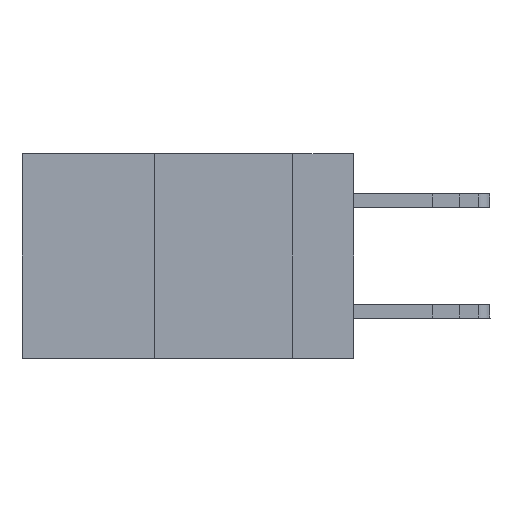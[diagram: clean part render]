
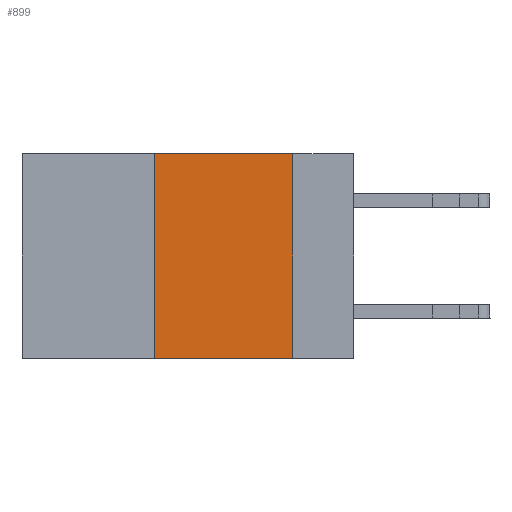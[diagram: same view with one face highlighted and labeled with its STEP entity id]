
A CAD part, left-side view. The second image highlights one B-rep face of the part: STEP entity #899.
In plain terms, the highlighted planar face has unit normal (-1, 0, 0).
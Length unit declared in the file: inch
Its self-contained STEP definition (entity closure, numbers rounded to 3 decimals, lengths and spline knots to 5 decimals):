
#395 = CARTESIAN_POINT ( 'NONE',  ( 0., 0.11, 0. ) ) ;
#654 = VERTEX_POINT ( 'NONE', #395 ) ;
#899 = ADVANCED_FACE ( 'NONE', ( #26525 ), #13610, .F. ) ;
#933 = EDGE_CURVE ( 'NONE', #654, #10693, #12890, .T. ) ;
#2144 = DIRECTION ( 'NONE',  ( 0., 0., -1. ) ) ;
#2252 = VERTEX_POINT ( 'NONE', #13262 ) ;
#3019 = LINE ( 'NONE', #32753, #29172 ) ;
#3644 = DIRECTION ( 'NONE',  ( 0., 0., 1. ) ) ;
#4279 = CARTESIAN_POINT ( 'NONE',  ( 0., 0.36, -0.37 ) ) ;
#5188 = CARTESIAN_POINT ( 'NONE',  ( 0., 0.6, 0. ) ) ;
#7033 = ORIENTED_EDGE ( 'NONE', *, *, #8444, .T. ) ;
#7741 = CARTESIAN_POINT ( 'NONE',  ( 0., 0.6, 0. ) ) ;
#8444 = EDGE_CURVE ( 'NONE', #27144, #10693, #3019, .T. ) ;
#10505 = ORIENTED_EDGE ( 'NONE', *, *, #12378, .F. ) ;
#10693 = VERTEX_POINT ( 'NONE', #13856 ) ;
#10860 = EDGE_LOOP ( 'NONE', ( #31472, #10505, #21145, #7033 ) ) ;
#11701 = VECTOR ( 'NONE', #23854, 39.37008 ) ;
#12378 = EDGE_CURVE ( 'NONE', #2252, #654, #34985, .T. ) ;
#12890 = LINE ( 'NONE', #32778, #11701 ) ;
#13262 = CARTESIAN_POINT ( 'NONE',  ( 0., 0.36, 0. ) ) ;
#13610 = PLANE ( 'NONE',  #32897 ) ;
#13856 = CARTESIAN_POINT ( 'NONE',  ( 0., 0.11, -0.37 ) ) ;
#14873 = VECTOR ( 'NONE', #3644, 39.37008 ) ;
#16986 = DIRECTION ( 'NONE',  ( 0., -1., 0. ) ) ;
#18664 = VECTOR ( 'NONE', #21375, 39.37008 ) ;
#21145 = ORIENTED_EDGE ( 'NONE', *, *, #31111, .F. ) ;
#21375 = DIRECTION ( 'NONE',  ( 0., -1., 0. ) ) ;
#23854 = DIRECTION ( 'NONE',  ( 0., 0., -1. ) ) ;
#26525 = FACE_OUTER_BOUND ( 'NONE', #10860, .T. ) ;
#27144 = VERTEX_POINT ( 'NONE', #4279 ) ;
#29172 = VECTOR ( 'NONE', #16986, 39.37008 ) ;
#29756 = DIRECTION ( 'NONE',  ( 1., 0., 0. ) ) ;
#31111 = EDGE_CURVE ( 'NONE', #27144, #2252, #33576, .T. ) ;
#31472 = ORIENTED_EDGE ( 'NONE', *, *, #933, .F. ) ;
#32753 = CARTESIAN_POINT ( 'NONE',  ( 0., 0.6, -0.37 ) ) ;
#32778 = CARTESIAN_POINT ( 'NONE',  ( 0., 0.11, 0. ) ) ;
#32897 = AXIS2_PLACEMENT_3D ( 'NONE', #5188, #29756, #2144 ) ;
#33576 = LINE ( 'NONE', #33760, #14873 ) ;
#33760 = CARTESIAN_POINT ( 'NONE',  ( 0., 0.36, 0. ) ) ;
#34985 = LINE ( 'NONE', #7741, #18664 ) ;
